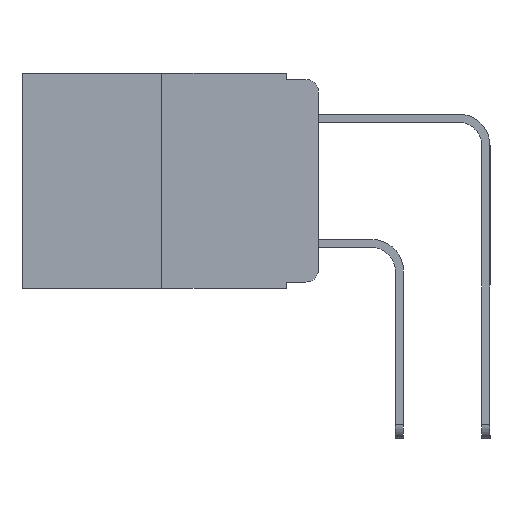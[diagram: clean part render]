
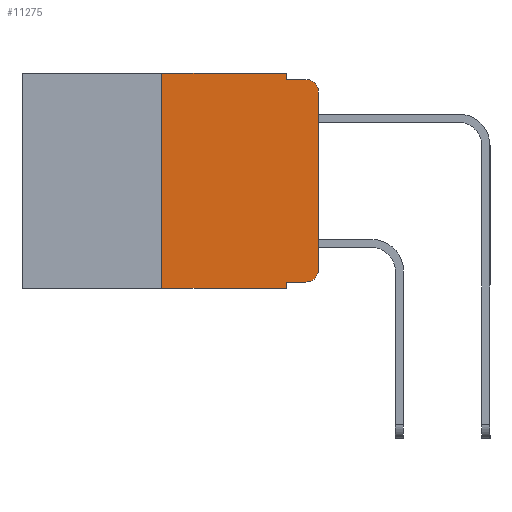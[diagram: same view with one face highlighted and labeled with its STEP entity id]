
A CAD part, left-side view. The second image highlights one B-rep face of the part: STEP entity #11275.
In plain terms, the highlighted planar face has unit normal (-1, 0, 0).
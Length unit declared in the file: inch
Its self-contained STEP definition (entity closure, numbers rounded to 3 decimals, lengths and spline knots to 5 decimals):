
#51 = CARTESIAN_POINT ( 'NONE',  ( 0., 0.051, 0. ) ) ;
#562 = VERTEX_POINT ( 'NONE', #7390 ) ;
#634 = CARTESIAN_POINT ( 'NONE',  ( 0., 0.051, 0. ) ) ;
#1278 = VERTEX_POINT ( 'NONE', #19728 ) ;
#1481 = DIRECTION ( 'NONE',  ( -1., 0., 0. ) ) ;
#1595 = CIRCLE ( 'NONE', #15560, 0.02 ) ;
#1820 = VECTOR ( 'NONE', #5596, 39.37008 ) ;
#2384 = EDGE_CURVE ( 'NONE', #1278, #13657, #12224, .T. ) ;
#3188 = VERTEX_POINT ( 'NONE', #11331 ) ;
#3196 = LINE ( 'NONE', #5722, #6989 ) ;
#3522 = VERTEX_POINT ( 'NONE', #13887 ) ;
#3909 = DIRECTION ( 'NONE',  ( 0., -1., 0. ) ) ;
#4120 = VECTOR ( 'NONE', #3909, 39.37008 ) ;
#4296 = DIRECTION ( 'NONE',  ( 0., -1., 0. ) ) ;
#4671 = AXIS2_PLACEMENT_3D ( 'NONE', #15125, #6218, #16577 ) ;
#5000 = DIRECTION ( 'NONE',  ( 0., -1., 0. ) ) ;
#5139 = DIRECTION ( 'NONE',  ( 0., 0., -1. ) ) ;
#5393 = VECTOR ( 'NONE', #10372, 39.37008 ) ;
#5579 = VERTEX_POINT ( 'NONE', #13577 ) ;
#5596 = DIRECTION ( 'NONE',  ( 0., 0., 1. ) ) ;
#5722 = CARTESIAN_POINT ( 'NONE',  ( 0., 0.051, -0.01 ) ) ;
#6218 = DIRECTION ( 'NONE',  ( -1., 0., 0. ) ) ;
#6222 = EDGE_CURVE ( 'NONE', #17459, #562, #14555, .T. ) ;
#6271 = VECTOR ( 'NONE', #9769, 39.37008 ) ;
#6719 = ORIENTED_EDGE ( 'NONE', *, *, #12276, .F. ) ;
#6989 = VECTOR ( 'NONE', #8821, 39.37008 ) ;
#7264 = EDGE_CURVE ( 'NONE', #5579, #17459, #19473, .T. ) ;
#7390 = CARTESIAN_POINT ( 'NONE',  ( 0., 0., -0.313 ) ) ;
#7684 = ORIENTED_EDGE ( 'NONE', *, *, #2384, .F. ) ;
#7884 = ORIENTED_EDGE ( 'NONE', *, *, #19651, .T. ) ;
#8294 = EDGE_CURVE ( 'NONE', #5579, #3188, #12230, .T. ) ;
#8772 = EDGE_LOOP ( 'NONE', ( #17111, #10284, #6719, #15070, #7684, #15543, #7884, #15738, #9011, #12328 ) ) ;
#8821 = DIRECTION ( 'NONE',  ( 0., -1., 0. ) ) ;
#8836 = LINE ( 'NONE', #16007, #1820 ) ;
#9000 = LINE ( 'NONE', #11910, #5393 ) ;
#9011 = ORIENTED_EDGE ( 'NONE', *, *, #7264, .T. ) ;
#9296 = EDGE_CURVE ( 'NONE', #3522, #1278, #9000, .T. ) ;
#9698 = DIRECTION ( 'NONE',  ( 0., 0., -1. ) ) ;
#9769 = DIRECTION ( 'NONE',  ( 0., 0., -1. ) ) ;
#9855 = LINE ( 'NONE', #14825, #12840 ) ;
#10262 = VERTEX_POINT ( 'NONE', #13156 ) ;
#10284 = ORIENTED_EDGE ( 'NONE', *, *, #13251, .T. ) ;
#10360 = VERTEX_POINT ( 'NONE', #10402 ) ;
#10372 = DIRECTION ( 'NONE',  ( 0., 0., 1. ) ) ;
#10402 = CARTESIAN_POINT ( 'NONE',  ( 0., 0.02, -0.01 ) ) ;
#10920 = CARTESIAN_POINT ( 'NONE',  ( 0., 0.02, -0.03 ) ) ;
#11275 = ADVANCED_FACE ( 'NONE', ( #14195 ), #12659, .F. ) ;
#11281 = EDGE_CURVE ( 'NONE', #13657, #16204, #18022, .T. ) ;
#11331 = CARTESIAN_POINT ( 'NONE',  ( 0., 0.051, -0.343 ) ) ;
#11910 = CARTESIAN_POINT ( 'NONE',  ( 0., 0.25, 0. ) ) ;
#12224 = LINE ( 'NONE', #17493, #19441 ) ;
#12230 = LINE ( 'NONE', #51, #15640 ) ;
#12276 = EDGE_CURVE ( 'NONE', #16204, #10360, #3196, .T. ) ;
#12328 = ORIENTED_EDGE ( 'NONE', *, *, #6222, .T. ) ;
#12408 = DIRECTION ( 'NONE',  ( 0., 0., -1. ) ) ;
#12659 = PLANE ( 'NONE',  #15787 ) ;
#12840 = VECTOR ( 'NONE', #4296, 39.37008 ) ;
#13156 = CARTESIAN_POINT ( 'NONE',  ( 0., 0., -0.03 ) ) ;
#13251 = EDGE_CURVE ( 'NONE', #10262, #10360, #1595, .T. ) ;
#13577 = CARTESIAN_POINT ( 'NONE',  ( 0., 0.051, -0.333 ) ) ;
#13657 = VERTEX_POINT ( 'NONE', #634 ) ;
#13887 = CARTESIAN_POINT ( 'NONE',  ( 0., 0.25, -0.343 ) ) ;
#14063 = CARTESIAN_POINT ( 'NONE',  ( 0., 0.473, 0. ) ) ;
#14121 = DIRECTION ( 'NONE',  ( 1., 0., 0. ) ) ;
#14195 = FACE_OUTER_BOUND ( 'NONE', #8772, .T. ) ;
#14221 = EDGE_CURVE ( 'NONE', #562, #10262, #8836, .T. ) ;
#14555 = CIRCLE ( 'NONE', #4671, 0.02 ) ;
#14825 = CARTESIAN_POINT ( 'NONE',  ( 0., 0.473, -0.343 ) ) ;
#15070 = ORIENTED_EDGE ( 'NONE', *, *, #11281, .F. ) ;
#15125 = CARTESIAN_POINT ( 'NONE',  ( 0., 0.02, -0.313 ) ) ;
#15543 = ORIENTED_EDGE ( 'NONE', *, *, #9296, .F. ) ;
#15560 = AXIS2_PLACEMENT_3D ( 'NONE', #10920, #1481, #12408 ) ;
#15589 = CARTESIAN_POINT ( 'NONE',  ( 0., 0.051, 0. ) ) ;
#15640 = VECTOR ( 'NONE', #9698, 39.37008 ) ;
#15738 = ORIENTED_EDGE ( 'NONE', *, *, #8294, .F. ) ;
#15787 = AXIS2_PLACEMENT_3D ( 'NONE', #14063, #14121, #5139 ) ;
#15885 = CARTESIAN_POINT ( 'NONE',  ( 0., 0.051, -0.01 ) ) ;
#15988 = CARTESIAN_POINT ( 'NONE',  ( 0., 0.051, -0.333 ) ) ;
#16007 = CARTESIAN_POINT ( 'NONE',  ( 0., 0., 0. ) ) ;
#16204 = VERTEX_POINT ( 'NONE', #15885 ) ;
#16577 = DIRECTION ( 'NONE',  ( 0., 0., -1. ) ) ;
#16586 = CARTESIAN_POINT ( 'NONE',  ( 0., 0.02, -0.333 ) ) ;
#17111 = ORIENTED_EDGE ( 'NONE', *, *, #14221, .T. ) ;
#17459 = VERTEX_POINT ( 'NONE', #16586 ) ;
#17493 = CARTESIAN_POINT ( 'NONE',  ( 0., 0.473, 0. ) ) ;
#18022 = LINE ( 'NONE', #15589, #6271 ) ;
#19441 = VECTOR ( 'NONE', #5000, 39.37008 ) ;
#19473 = LINE ( 'NONE', #15988, #4120 ) ;
#19651 = EDGE_CURVE ( 'NONE', #3522, #3188, #9855, .T. ) ;
#19728 = CARTESIAN_POINT ( 'NONE',  ( 0., 0.25, 0. ) ) ;
